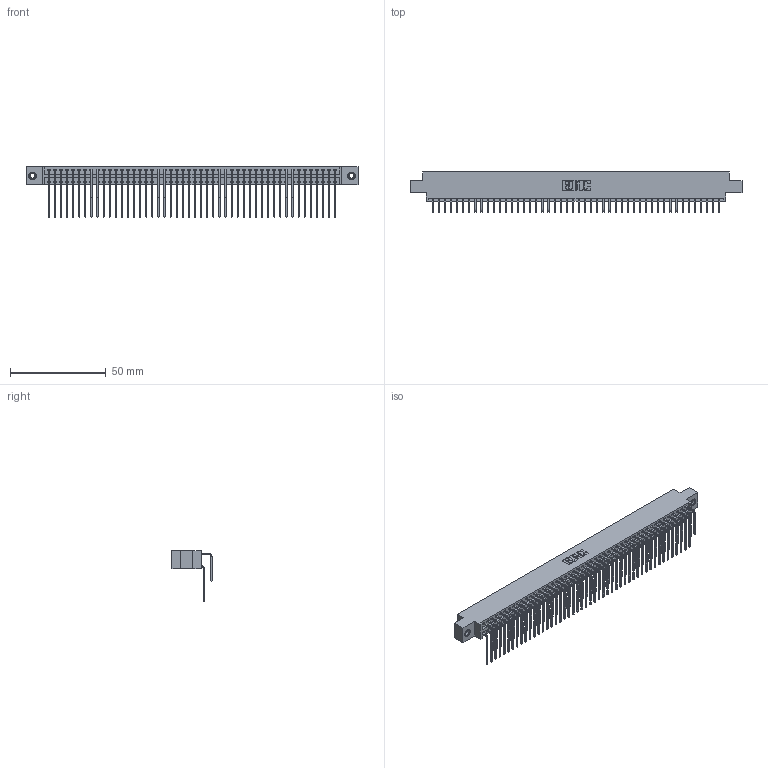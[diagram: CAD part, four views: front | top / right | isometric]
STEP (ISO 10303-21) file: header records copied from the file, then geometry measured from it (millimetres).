
FILE_DESCRIPTION (( 'STEP AP203' ), '1' );
FILE_NAME ('346-096-559-807.STEP', '2018-08-30T07:52:26', ( '' ), ( '' ), 'SwSTEP 2.0', 'SolidWorks 2016', '' );
FILE_SCHEMA (( 'CONFIG_CONTROL_DESIGN' ));
Length unit declared in the file: inch
Products named in the file (5): 346 Part_0.170 Offset - 0.156 Dia-TI; 345-292-001_558 559 Tail - 1; 345-292-001_559 Tail - 2; 345-250-001_345-250-005-103; 346-096-559-807
Assembly tree (99 placements, depth 2):
  346-096-559-807
    346 Part_0.170 Offset - 0.156 Dia-TI
    345-292-001_558 559 Tail - 1  x48
    345-292-001_559 Tail - 2  x48
    345-250-001_345-250-005-103  x2
Bounding box: 172.97 x 20.89 x 26.16 mm (x, y, z)
Volume: 17299.4 mm3; surface area: 26743.6 mm2
Topology: 99 solids, 99 shells, 5370 faces, 15933 edges, 10486 vertices
Faces by surface type: plane 3664, cylinder 1690, cone 12, torus 4
Entity records: 33620 total; most frequent: CARTESIAN_POINT 5570, ORIENTED_EDGE 5446, DIRECTION 4957, EDGE_CURVE 2723, LINE 2339, VECTOR 2339, VERTEX_POINT 1808, AXIS2_PLACEMENT_3D 1309
